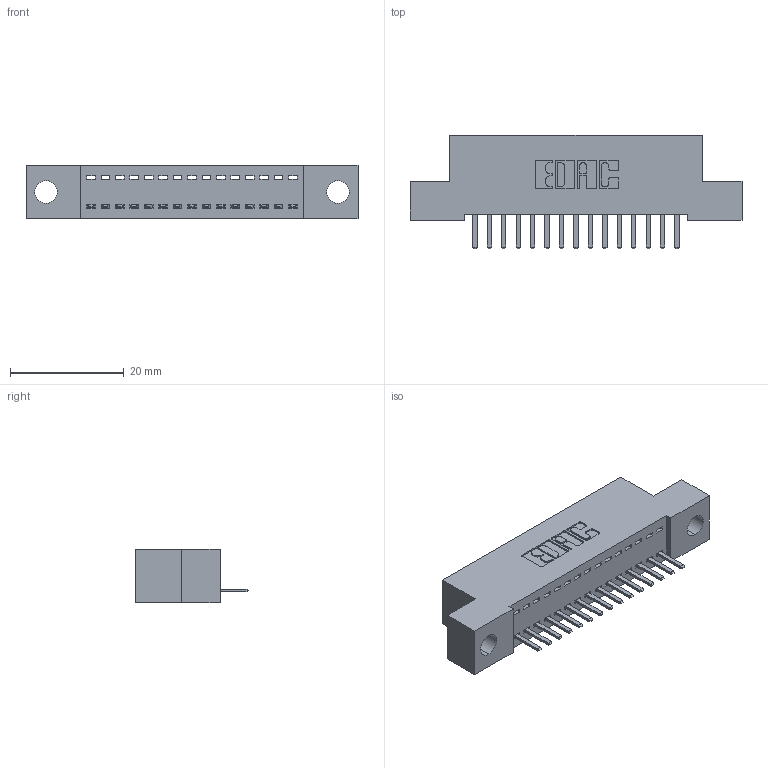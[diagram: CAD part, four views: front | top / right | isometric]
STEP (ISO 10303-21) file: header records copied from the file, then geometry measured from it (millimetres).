
FILE_DESCRIPTION (( 'STEP AP203' ), '1' );
FILE_NAME ('342-015-520-104.STEP', '2018-08-10T18:47:24', ( '' ), ( '' ), 'SwSTEP 2.0', 'SolidWorks 2016', '' );
FILE_SCHEMA (( 'CONFIG_CONTROL_DESIGN' ));
Length unit declared in the file: inch
Products named in the file (3): 342-015-520-104; 342 Part_.156 TH; 345-292-001_345-293-120
Assembly tree (16 placements, depth 2):
  342-015-520-104
    342 Part_.156 TH
    345-292-001_345-293-120  x15
Bounding box: 58.42 x 20.02 x 9.4 mm (x, y, z)
Volume: 4892.6 mm3; surface area: 6361.3 mm2
Topology: 16 solids, 16 shells, 1040 faces, 3059 edges, 1998 vertices
Faces by surface type: plane 726, cylinder 314
Entity records: 12647 total; most frequent: CARTESIAN_POINT 2203, ORIENTED_EDGE 2142, DIRECTION 1901, EDGE_CURVE 1071, VECTOR 939, LINE 939, VERTEX_POINT 710, AXIS2_PLACEMENT_3D 481
